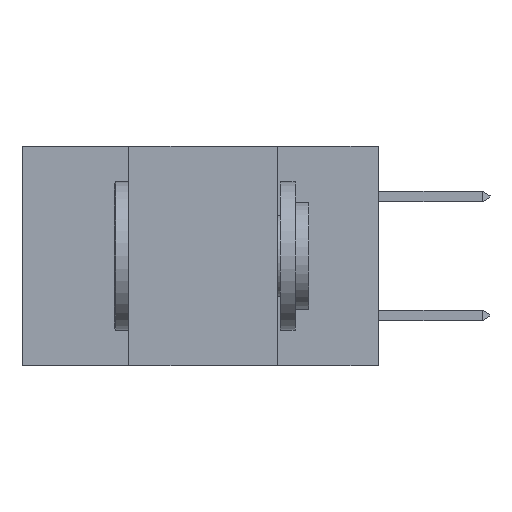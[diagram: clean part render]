
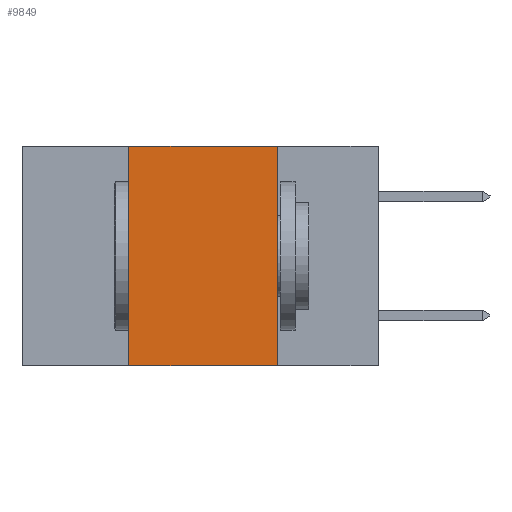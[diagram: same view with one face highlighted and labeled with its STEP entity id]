
A CAD part, left-side view. The second image highlights one B-rep face of the part: STEP entity #9849.
In plain terms, the highlighted planar face has unit normal (-1, 0, 0).
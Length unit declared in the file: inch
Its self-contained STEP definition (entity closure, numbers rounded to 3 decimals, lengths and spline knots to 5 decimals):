
#468 = ORIENTED_EDGE ( 'NONE', *, *, #13480, .F. ) ;
#773 = VERTEX_POINT ( 'NONE', #10608 ) ;
#964 = EDGE_CURVE ( 'NONE', #6961, #13354, #12391, .T. ) ;
#1944 = DIRECTION ( 'NONE',  ( 1., 0., 0. ) ) ;
#2021 = FACE_OUTER_BOUND ( 'NONE', #5726, .T. ) ;
#2174 = ORIENTED_EDGE ( 'NONE', *, *, #12359, .F. ) ;
#2393 = DIRECTION ( 'NONE',  ( 0., 0., 1. ) ) ;
#2443 = VECTOR ( 'NONE', #2393, 39.37008 ) ;
#2578 = VECTOR ( 'NONE', #3989, 39.37008 ) ;
#2606 = DIRECTION ( 'NONE',  ( 0., 0., -1. ) ) ;
#3916 = LINE ( 'NONE', #8993, #8694 ) ;
#3989 = DIRECTION ( 'NONE',  ( 0., -1., 0. ) ) ;
#4237 = CARTESIAN_POINT ( 'NONE',  ( 0., 0.6, 0. ) ) ;
#4343 = VECTOR ( 'NONE', #10027, 39.37008 ) ;
#5294 = ORIENTED_EDGE ( 'NONE', *, *, #6605, .T. ) ;
#5726 = EDGE_LOOP ( 'NONE', ( #468, #11133, #2174, #5294 ) ) ;
#6605 = EDGE_CURVE ( 'NONE', #13610, #773, #12807, .T. ) ;
#6961 = VERTEX_POINT ( 'NONE', #15094 ) ;
#8694 = VECTOR ( 'NONE', #2606, 39.37008 ) ;
#8993 = CARTESIAN_POINT ( 'NONE',  ( 0., 0.17, -0.37 ) ) ;
#9849 = ADVANCED_FACE ( 'NONE', ( #2021 ), #11984, .F. ) ;
#10027 = DIRECTION ( 'NONE',  ( 0., -1., 0. ) ) ;
#10507 = LINE ( 'NONE', #15484, #2443 ) ;
#10608 = CARTESIAN_POINT ( 'NONE',  ( 0., 0.17, -0.37 ) ) ;
#11006 = AXIS2_PLACEMENT_3D ( 'NONE', #4237, #1944, #15356 ) ;
#11133 = ORIENTED_EDGE ( 'NONE', *, *, #964, .F. ) ;
#11667 = CARTESIAN_POINT ( 'NONE',  ( 0., 0.42, -0.37 ) ) ;
#11984 = PLANE ( 'NONE',  #11006 ) ;
#12359 = EDGE_CURVE ( 'NONE', #13610, #6961, #10507, .T. ) ;
#12391 = LINE ( 'NONE', #16056, #4343 ) ;
#12807 = LINE ( 'NONE', #15197, #2578 ) ;
#13354 = VERTEX_POINT ( 'NONE', #13470 ) ;
#13470 = CARTESIAN_POINT ( 'NONE',  ( 0., 0.17, 0. ) ) ;
#13480 = EDGE_CURVE ( 'NONE', #13354, #773, #3916, .T. ) ;
#13610 = VERTEX_POINT ( 'NONE', #11667 ) ;
#15094 = CARTESIAN_POINT ( 'NONE',  ( 0., 0.42, 0. ) ) ;
#15197 = CARTESIAN_POINT ( 'NONE',  ( 0., 0.6, -0.37 ) ) ;
#15356 = DIRECTION ( 'NONE',  ( 0., 0., -1. ) ) ;
#15484 = CARTESIAN_POINT ( 'NONE',  ( 0., 0.42, -0.37 ) ) ;
#16056 = CARTESIAN_POINT ( 'NONE',  ( 0., 0.6, 0. ) ) ;
